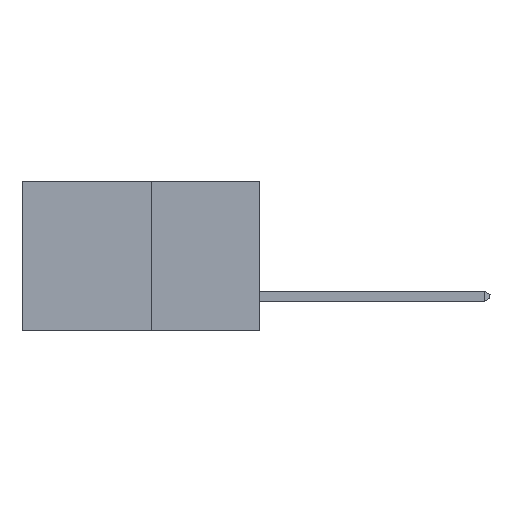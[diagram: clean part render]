
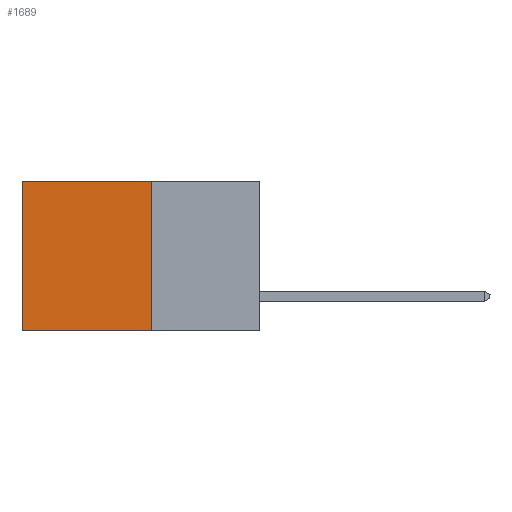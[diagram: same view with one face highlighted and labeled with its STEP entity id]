
A CAD part, left-side view. The second image highlights one B-rep face of the part: STEP entity #1689.
In plain terms, the highlighted planar face has unit normal (-1, 0, 0).
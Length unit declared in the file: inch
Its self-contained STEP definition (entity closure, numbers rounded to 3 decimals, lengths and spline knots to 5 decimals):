
#357 = CARTESIAN_POINT ( 'NONE',  ( 0.277, 0.27, 0. ) ) ;
#387 = DIRECTION ( 'NONE',  ( 0., 1., 0. ) ) ;
#1161 = DIRECTION ( 'NONE',  ( 1., 0., 0. ) ) ;
#1538 = VECTOR ( 'NONE', #6745, 39.37008 ) ;
#1689 = ADVANCED_FACE ( 'NONE', ( #12193 ), #12304, .F. ) ;
#2327 = CARTESIAN_POINT ( 'NONE',  ( 0.277, 0.27, -0.37 ) ) ;
#2569 = DIRECTION ( 'NONE',  ( 0., 0., -1. ) ) ;
#2626 = LINE ( 'NONE', #357, #5317 ) ;
#2695 = AXIS2_PLACEMENT_3D ( 'NONE', #6124, #1161, #2569 ) ;
#3060 = CARTESIAN_POINT ( 'NONE',  ( 0.277, 0.59, -0.37 ) ) ;
#3351 = DIRECTION ( 'NONE',  ( 0., 1., 0. ) ) ;
#3431 = EDGE_LOOP ( 'NONE', ( #5183, #5232, #5242, #5255 ) ) ;
#3869 = EDGE_CURVE ( 'NONE', #5227, #9552, #12237, .T. ) ;
#4525 = EDGE_CURVE ( 'NONE', #5227, #6195, #2626, .T. ) ;
#4572 = VECTOR ( 'NONE', #3351, 39.37008 ) ;
#4617 = DIRECTION ( 'NONE',  ( 0., 0., -1. ) ) ;
#4692 = CARTESIAN_POINT ( 'NONE',  ( 0.277, 0.27, -0.37 ) ) ;
#4882 = VECTOR ( 'NONE', #4617, 39.37008 ) ;
#5183 = ORIENTED_EDGE ( 'NONE', *, *, #7332, .T. ) ;
#5227 = VERTEX_POINT ( 'NONE', #7898 ) ;
#5232 = ORIENTED_EDGE ( 'NONE', *, *, #11207, .F. ) ;
#5242 = ORIENTED_EDGE ( 'NONE', *, *, #3869, .F. ) ;
#5255 = ORIENTED_EDGE ( 'NONE', *, *, #4525, .T. ) ;
#5317 = VECTOR ( 'NONE', #387, 39.37008 ) ;
#6124 = CARTESIAN_POINT ( 'NONE',  ( 0.277, 0.27, -0.37 ) ) ;
#6195 = VERTEX_POINT ( 'NONE', #9006 ) ;
#6567 = LINE ( 'NONE', #11542, #1538 ) ;
#6716 = VERTEX_POINT ( 'NONE', #3060 ) ;
#6745 = DIRECTION ( 'NONE',  ( 0., 0., -1. ) ) ;
#6803 = CARTESIAN_POINT ( 'NONE',  ( 0.277, 0.27, -0.37 ) ) ;
#7187 = LINE ( 'NONE', #2327, #4572 ) ;
#7332 = EDGE_CURVE ( 'NONE', #6195, #6716, #6567, .T. ) ;
#7898 = CARTESIAN_POINT ( 'NONE',  ( 0.277, 0.27, 0. ) ) ;
#9006 = CARTESIAN_POINT ( 'NONE',  ( 0.277, 0.59, 0. ) ) ;
#9552 = VERTEX_POINT ( 'NONE', #6803 ) ;
#11207 = EDGE_CURVE ( 'NONE', #9552, #6716, #7187, .T. ) ;
#11542 = CARTESIAN_POINT ( 'NONE',  ( 0.277, 0.59, -0.37 ) ) ;
#12193 = FACE_OUTER_BOUND ( 'NONE', #3431, .T. ) ;
#12237 = LINE ( 'NONE', #4692, #4882 ) ;
#12304 = PLANE ( 'NONE',  #2695 ) ;
